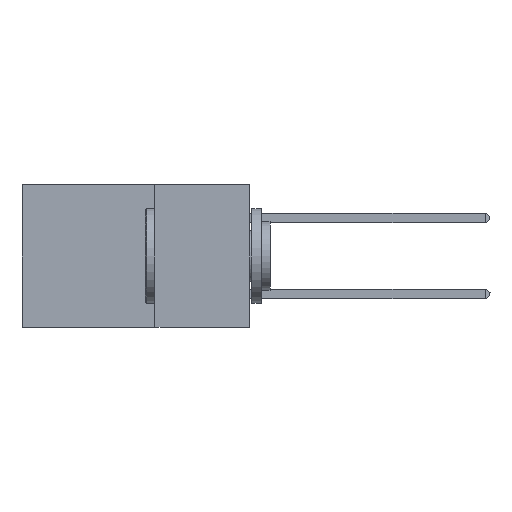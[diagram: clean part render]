
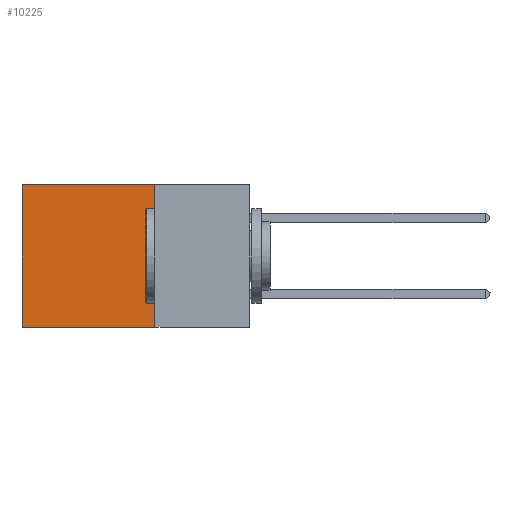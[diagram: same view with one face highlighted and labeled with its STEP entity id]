
A CAD part, left-side view. The second image highlights one B-rep face of the part: STEP entity #10225.
In plain terms, the highlighted planar face has unit normal (-1, 0, 0).
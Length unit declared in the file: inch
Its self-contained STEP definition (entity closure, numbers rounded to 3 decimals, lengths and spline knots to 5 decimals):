
#24 = DIRECTION ( 'NONE',  ( 1., 0., 0. ) ) ;
#1447 = LINE ( 'NONE', #4063, #11565 ) ;
#1550 = CARTESIAN_POINT ( 'NONE',  ( 0.2875, 0.25, -0.375 ) ) ;
#2059 = EDGE_CURVE ( 'NONE', #12170, #6456, #1447, .T. ) ;
#2491 = ORIENTED_EDGE ( 'NONE', *, *, #15921, .F. ) ;
#2869 = CARTESIAN_POINT ( 'NONE',  ( 0.2875, 0.25, -0.375 ) ) ;
#3750 = PLANE ( 'NONE',  #13785 ) ;
#4063 = CARTESIAN_POINT ( 'NONE',  ( 0.2875, 0.25, 0. ) ) ;
#5347 = DIRECTION ( 'NONE',  ( 0., 1., 0. ) ) ;
#6456 = VERTEX_POINT ( 'NONE', #13823 ) ;
#6468 = DIRECTION ( 'NONE',  ( 0., 1., 0. ) ) ;
#7372 = LINE ( 'NONE', #8568, #9563 ) ;
#7601 = DIRECTION ( 'NONE',  ( 0., 0., -1. ) ) ;
#8567 = VECTOR ( 'NONE', #10532, 39.37008 ) ;
#8568 = CARTESIAN_POINT ( 'NONE',  ( 0.2875, 0.6, -0.375 ) ) ;
#8623 = VERTEX_POINT ( 'NONE', #9306 ) ;
#8761 = LINE ( 'NONE', #1550, #8567 ) ;
#8996 = ORIENTED_EDGE ( 'NONE', *, *, #15943, .F. ) ;
#9306 = CARTESIAN_POINT ( 'NONE',  ( 0.2875, 0.6, -0.375 ) ) ;
#9563 = VECTOR ( 'NONE', #7601, 39.37008 ) ;
#10084 = DIRECTION ( 'NONE',  ( 0., 0., -1. ) ) ;
#10225 = ADVANCED_FACE ( 'NONE', ( #13120 ), #3750, .F. ) ;
#10532 = DIRECTION ( 'NONE',  ( 0., 0., -1. ) ) ;
#11565 = VECTOR ( 'NONE', #5347, 39.37008 ) ;
#11690 = ORIENTED_EDGE ( 'NONE', *, *, #2059, .T. ) ;
#12061 = EDGE_LOOP ( 'NONE', ( #12791, #2491, #8996, #11690 ) ) ;
#12170 = VERTEX_POINT ( 'NONE', #14209 ) ;
#12609 = CARTESIAN_POINT ( 'NONE',  ( 0.2875, 0.25, -0.375 ) ) ;
#12615 = CARTESIAN_POINT ( 'NONE',  ( 0.2875, 0.25, -0.375 ) ) ;
#12791 = ORIENTED_EDGE ( 'NONE', *, *, #14949, .T. ) ;
#13120 = FACE_OUTER_BOUND ( 'NONE', #12061, .T. ) ;
#13785 = AXIS2_PLACEMENT_3D ( 'NONE', #12609, #24, #10084 ) ;
#13823 = CARTESIAN_POINT ( 'NONE',  ( 0.2875, 0.6, 0. ) ) ;
#14075 = LINE ( 'NONE', #2869, #14876 ) ;
#14209 = CARTESIAN_POINT ( 'NONE',  ( 0.2875, 0.25, 0. ) ) ;
#14876 = VECTOR ( 'NONE', #6468, 39.37008 ) ;
#14949 = EDGE_CURVE ( 'NONE', #6456, #8623, #7372, .T. ) ;
#15808 = VERTEX_POINT ( 'NONE', #12615 ) ;
#15921 = EDGE_CURVE ( 'NONE', #15808, #8623, #14075, .T. ) ;
#15943 = EDGE_CURVE ( 'NONE', #12170, #15808, #8761, .T. ) ;
